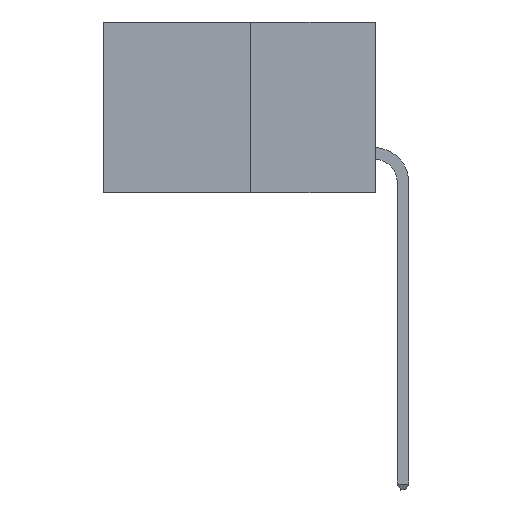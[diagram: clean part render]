
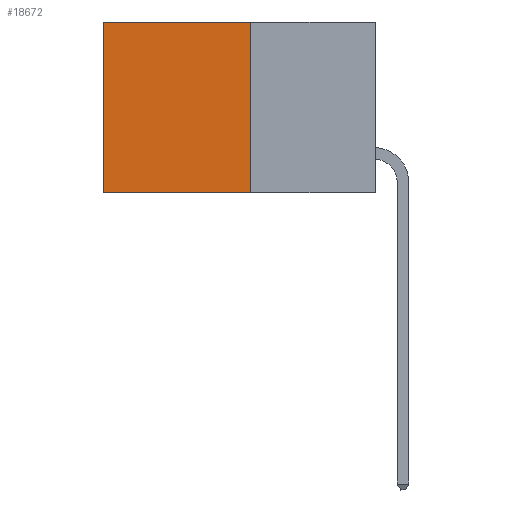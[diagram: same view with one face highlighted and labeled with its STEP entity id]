
A CAD part, left-side view. The second image highlights one B-rep face of the part: STEP entity #18672.
In plain terms, the highlighted planar face has unit normal (-1, 0, 0).
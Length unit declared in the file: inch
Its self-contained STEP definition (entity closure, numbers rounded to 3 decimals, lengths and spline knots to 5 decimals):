
#1063 = AXIS2_PLACEMENT_3D ( 'NONE', #23895, #10062, #26264 ) ;
#1356 = DIRECTION ( 'NONE',  ( 0., 1., 0. ) ) ;
#1723 = CARTESIAN_POINT ( 'NONE',  ( 0.277, 0.59, -0.37 ) ) ;
#1728 = CARTESIAN_POINT ( 'NONE',  ( 0.277, 0.27, -0.37 ) ) ;
#1782 = VERTEX_POINT ( 'NONE', #1728 ) ;
#2118 = EDGE_LOOP ( 'NONE', ( #29726, #3011, #12921, #7350 ) ) ;
#2635 = VERTEX_POINT ( 'NONE', #17696 ) ;
#3011 = ORIENTED_EDGE ( 'NONE', *, *, #5095, .F. ) ;
#3328 = VECTOR ( 'NONE', #1356, 39.37008 ) ;
#3820 = CARTESIAN_POINT ( 'NONE',  ( 0.277, 0.27, 0. ) ) ;
#4005 = EDGE_CURVE ( 'NONE', #2635, #25444, #11812, .T. ) ;
#5095 = EDGE_CURVE ( 'NONE', #1782, #25444, #9520, .T. ) ;
#5461 = CARTESIAN_POINT ( 'NONE',  ( 0.277, 0.27, 0. ) ) ;
#6098 = LINE ( 'NONE', #8971, #17746 ) ;
#7093 = CARTESIAN_POINT ( 'NONE',  ( 0.277, 0.27, -0.37 ) ) ;
#7350 = ORIENTED_EDGE ( 'NONE', *, *, #23480, .T. ) ;
#8208 = EDGE_CURVE ( 'NONE', #11930, #1782, #6098, .T. ) ;
#8971 = CARTESIAN_POINT ( 'NONE',  ( 0.277, 0.27, -0.37 ) ) ;
#9062 = DIRECTION ( 'NONE',  ( 0., 0., -1. ) ) ;
#9520 = LINE ( 'NONE', #7093, #3328 ) ;
#10062 = DIRECTION ( 'NONE',  ( 1., 0., 0. ) ) ;
#11130 = LINE ( 'NONE', #3820, #23389 ) ;
#11812 = LINE ( 'NONE', #27527, #23340 ) ;
#11930 = VERTEX_POINT ( 'NONE', #5461 ) ;
#12921 = ORIENTED_EDGE ( 'NONE', *, *, #8208, .F. ) ;
#17696 = CARTESIAN_POINT ( 'NONE',  ( 0.277, 0.59, 0. ) ) ;
#17746 = VECTOR ( 'NONE', #9062, 39.37008 ) ;
#18672 = ADVANCED_FACE ( 'NONE', ( #24798 ), #19215, .F. ) ;
#19215 = PLANE ( 'NONE',  #1063 ) ;
#19984 = DIRECTION ( 'NONE',  ( 0., 1., 0. ) ) ;
#23340 = VECTOR ( 'NONE', #30210, 39.37008 ) ;
#23389 = VECTOR ( 'NONE', #19984, 39.37008 ) ;
#23480 = EDGE_CURVE ( 'NONE', #11930, #2635, #11130, .T. ) ;
#23895 = CARTESIAN_POINT ( 'NONE',  ( 0.277, 0.27, -0.37 ) ) ;
#24798 = FACE_OUTER_BOUND ( 'NONE', #2118, .T. ) ;
#25444 = VERTEX_POINT ( 'NONE', #1723 ) ;
#26264 = DIRECTION ( 'NONE',  ( 0., 0., -1. ) ) ;
#27527 = CARTESIAN_POINT ( 'NONE',  ( 0.277, 0.59, -0.37 ) ) ;
#29726 = ORIENTED_EDGE ( 'NONE', *, *, #4005, .T. ) ;
#30210 = DIRECTION ( 'NONE',  ( 0., 0., -1. ) ) ;
